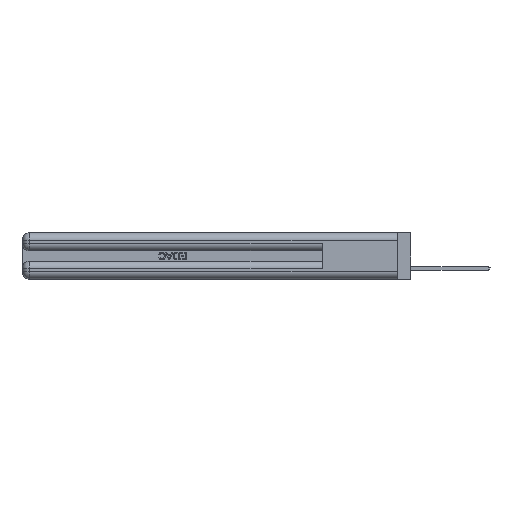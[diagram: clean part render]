
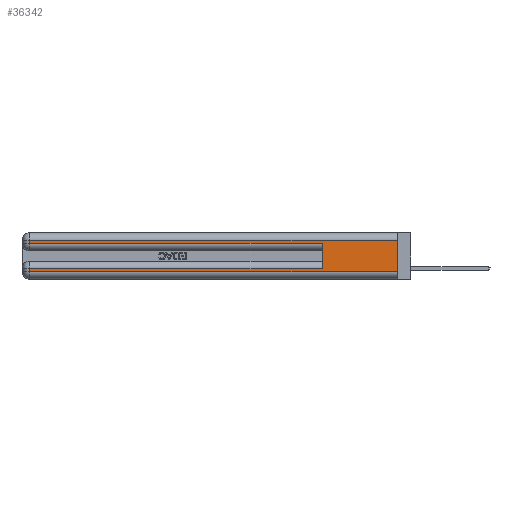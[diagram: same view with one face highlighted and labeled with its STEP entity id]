
A CAD part, left-side view. The second image highlights one B-rep face of the part: STEP entity #36342.
In plain terms, the highlighted planar face has unit normal (-1, 0, 0).
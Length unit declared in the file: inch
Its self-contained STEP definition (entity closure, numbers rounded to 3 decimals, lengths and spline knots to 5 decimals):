
#739 = LINE ( 'NONE', #44052, #32655 ) ;
#927 = VECTOR ( 'NONE', #1924, 39.37008 ) ;
#976 = CARTESIAN_POINT ( 'NONE',  ( 0., 2.94, 0.285 ) ) ;
#1078 = VECTOR ( 'NONE', #23221, 39.37008 ) ;
#1690 = DIRECTION ( 'NONE',  ( 0., 1., 0. ) ) ;
#1885 = VERTEX_POINT ( 'NONE', #53997 ) ;
#1924 = DIRECTION ( 'NONE',  ( 0., -1., 0. ) ) ;
#6238 = ORIENTED_EDGE ( 'NONE', *, *, #49935, .T. ) ;
#6281 = CARTESIAN_POINT ( 'NONE',  ( 0., 0., 0.31 ) ) ;
#6613 = CARTESIAN_POINT ( 'NONE',  ( 0., 0., 0.285 ) ) ;
#6661 = VERTEX_POINT ( 'NONE', #45239 ) ;
#6733 = LINE ( 'NONE', #28387, #29208 ) ;
#7496 = VECTOR ( 'NONE', #12960, 39.37008 ) ;
#12367 = VECTOR ( 'NONE', #48097, 39.37008 ) ;
#12960 = DIRECTION ( 'NONE',  ( 0., 0., 1. ) ) ;
#13464 = VERTEX_POINT ( 'NONE', #976 ) ;
#14399 = DIRECTION ( 'NONE',  ( 0., 0., -1. ) ) ;
#14813 = LINE ( 'NONE', #6613, #17456 ) ;
#15721 = DIRECTION ( 'NONE',  ( 0., -1., 0. ) ) ;
#15897 = DIRECTION ( 'NONE',  ( 0., 0., -1. ) ) ;
#15933 = ORIENTED_EDGE ( 'NONE', *, *, #42421, .F. ) ;
#16178 = VERTEX_POINT ( 'NONE', #46262 ) ;
#16300 = ORIENTED_EDGE ( 'NONE', *, *, #39897, .T. ) ;
#17456 = VECTOR ( 'NONE', #15721, 39.37008 ) ;
#18121 = ORIENTED_EDGE ( 'NONE', *, *, #19557, .T. ) ;
#18680 = LINE ( 'NONE', #25293, #7496 ) ;
#19557 = EDGE_CURVE ( 'NONE', #29378, #16178, #6733, .T. ) ;
#19857 = EDGE_CURVE ( 'NONE', #6661, #29378, #51755, .T. ) ;
#22123 = CARTESIAN_POINT ( 'NONE',  ( 0., 0., 0.37 ) ) ;
#22909 = DIRECTION ( 'NONE',  ( 0., 0., -1. ) ) ;
#23221 = DIRECTION ( 'NONE',  ( 0., 0., -1. ) ) ;
#23506 = ORIENTED_EDGE ( 'NONE', *, *, #33674, .T. ) ;
#25293 = CARTESIAN_POINT ( 'NONE',  ( 0., 0.6, 0.145 ) ) ;
#26682 = CARTESIAN_POINT ( 'NONE',  ( 0., 0., 0.37 ) ) ;
#28387 = CARTESIAN_POINT ( 'NONE',  ( 0., 2.94, 0.37 ) ) ;
#29208 = VECTOR ( 'NONE', #15897, 39.37008 ) ;
#29378 = VERTEX_POINT ( 'NONE', #38609 ) ;
#30601 = DIRECTION ( 'NONE',  ( 1., 0., 0. ) ) ;
#31355 = CARTESIAN_POINT ( 'NONE',  ( 0., 0., 0.06 ) ) ;
#32339 = EDGE_CURVE ( 'NONE', #43406, #1885, #53513, .T. ) ;
#32655 = VECTOR ( 'NONE', #22909, 39.37008 ) ;
#33118 = ORIENTED_EDGE ( 'NONE', *, *, #19857, .T. ) ;
#33445 = CARTESIAN_POINT ( 'NONE',  ( 0., 2.94, 0.31 ) ) ;
#33674 = EDGE_CURVE ( 'NONE', #43406, #36804, #54705, .T. ) ;
#35034 = PLANE ( 'NONE',  #52909 ) ;
#36342 = ADVANCED_FACE ( 'NONE', ( #45217 ), #35034, .F. ) ;
#36804 = VERTEX_POINT ( 'NONE', #33445 ) ;
#37479 = LINE ( 'NONE', #31355, #927 ) ;
#38609 = CARTESIAN_POINT ( 'NONE',  ( 0., 2.94, 0.085 ) ) ;
#39159 = ORIENTED_EDGE ( 'NONE', *, *, #49104, .T. ) ;
#39897 = EDGE_CURVE ( 'NONE', #16178, #1885, #37479, .T. ) ;
#41742 = CARTESIAN_POINT ( 'NONE',  ( 0., 0.6, 0.285 ) ) ;
#42136 = ORIENTED_EDGE ( 'NONE', *, *, #32339, .F. ) ;
#42421 = EDGE_CURVE ( 'NONE', #6661, #45149, #18680, .T. ) ;
#42516 = VECTOR ( 'NONE', #1690, 39.37008 ) ;
#43406 = VERTEX_POINT ( 'NONE', #52595 ) ;
#44052 = CARTESIAN_POINT ( 'NONE',  ( 0., 2.94, 0.37 ) ) ;
#45149 = VERTEX_POINT ( 'NONE', #41742 ) ;
#45217 = FACE_OUTER_BOUND ( 'NONE', #52086, .T. ) ;
#45239 = CARTESIAN_POINT ( 'NONE',  ( 0., 0.6, 0.085 ) ) ;
#46262 = CARTESIAN_POINT ( 'NONE',  ( 0., 2.94, 0.06 ) ) ;
#48097 = DIRECTION ( 'NONE',  ( 0., 1., 0. ) ) ;
#49104 = EDGE_CURVE ( 'NONE', #13464, #45149, #14813, .T. ) ;
#49935 = EDGE_CURVE ( 'NONE', #36804, #13464, #739, .T. ) ;
#51755 = LINE ( 'NONE', #52443, #42516 ) ;
#52086 = EDGE_LOOP ( 'NONE', ( #42136, #23506, #6238, #39159, #15933, #33118, #18121, #16300 ) ) ;
#52443 = CARTESIAN_POINT ( 'NONE',  ( 0., 0., 0.085 ) ) ;
#52595 = CARTESIAN_POINT ( 'NONE',  ( 0., 0., 0.31 ) ) ;
#52909 = AXIS2_PLACEMENT_3D ( 'NONE', #22123, #30601, #14399 ) ;
#53513 = LINE ( 'NONE', #26682, #1078 ) ;
#53997 = CARTESIAN_POINT ( 'NONE',  ( 0., 0., 0.06 ) ) ;
#54705 = LINE ( 'NONE', #6281, #12367 ) ;
